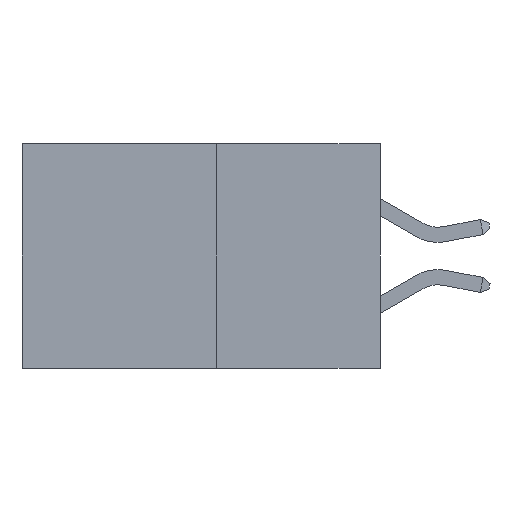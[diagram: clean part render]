
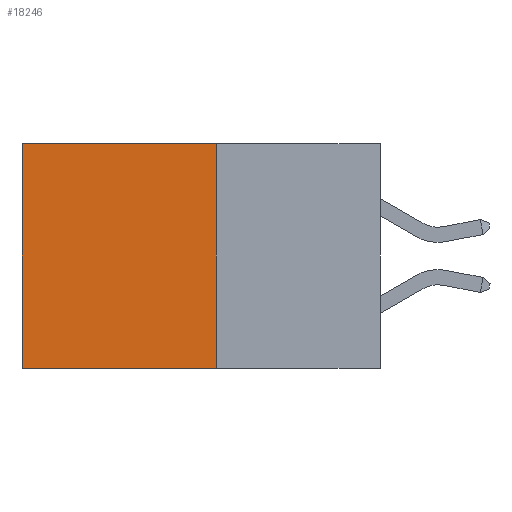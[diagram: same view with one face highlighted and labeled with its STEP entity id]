
A CAD part, left-side view. The second image highlights one B-rep face of the part: STEP entity #18246.
In plain terms, the highlighted planar face has unit normal (-1, 0, 0).
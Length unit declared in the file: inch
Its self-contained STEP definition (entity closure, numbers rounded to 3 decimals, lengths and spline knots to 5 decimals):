
#338 = CARTESIAN_POINT ( 'NONE',  ( 0.277, 0.27, -0.37 ) ) ;
#500 = CARTESIAN_POINT ( 'NONE',  ( 0.277, 0.27, 0. ) ) ;
#790 = VERTEX_POINT ( 'NONE', #1906 ) ;
#957 = EDGE_CURVE ( 'NONE', #18103, #5772, #1752, .T. ) ;
#1347 = ORIENTED_EDGE ( 'NONE', *, *, #20250, .T. ) ;
#1752 = LINE ( 'NONE', #20085, #15234 ) ;
#1906 = CARTESIAN_POINT ( 'NONE',  ( 0.277, 0.59, 0. ) ) ;
#2418 = EDGE_CURVE ( 'NONE', #790, #13445, #4125, .T. ) ;
#2867 = DIRECTION ( 'NONE',  ( 0., 1., 0. ) ) ;
#2894 = ORIENTED_EDGE ( 'NONE', *, *, #2418, .T. ) ;
#4125 = LINE ( 'NONE', #16833, #8122 ) ;
#4263 = DIRECTION ( 'NONE',  ( 1., 0., 0. ) ) ;
#5726 = CARTESIAN_POINT ( 'NONE',  ( 0.277, 0.59, -0.37 ) ) ;
#5772 = VERTEX_POINT ( 'NONE', #12422 ) ;
#5781 = ORIENTED_EDGE ( 'NONE', *, *, #957, .F. ) ;
#6367 = LINE ( 'NONE', #11327, #10371 ) ;
#6888 = DIRECTION ( 'NONE',  ( 0., 0., -1. ) ) ;
#7282 = FACE_OUTER_BOUND ( 'NONE', #9623, .T. ) ;
#8122 = VECTOR ( 'NONE', #15710, 39.37008 ) ;
#9623 = EDGE_LOOP ( 'NONE', ( #2894, #12051, #5781, #1347 ) ) ;
#9779 = EDGE_CURVE ( 'NONE', #5772, #13445, #17468, .T. ) ;
#10371 = VECTOR ( 'NONE', #2867, 39.37008 ) ;
#11028 = PLANE ( 'NONE',  #14331 ) ;
#11327 = CARTESIAN_POINT ( 'NONE',  ( 0.277, 0.27, 0. ) ) ;
#12051 = ORIENTED_EDGE ( 'NONE', *, *, #9779, .F. ) ;
#12422 = CARTESIAN_POINT ( 'NONE',  ( 0.277, 0.27, -0.37 ) ) ;
#13025 = VECTOR ( 'NONE', #15530, 39.37008 ) ;
#13445 = VERTEX_POINT ( 'NONE', #5726 ) ;
#14331 = AXIS2_PLACEMENT_3D ( 'NONE', #14394, #4263, #16062 ) ;
#14394 = CARTESIAN_POINT ( 'NONE',  ( 0.277, 0.27, -0.37 ) ) ;
#15234 = VECTOR ( 'NONE', #6888, 39.37008 ) ;
#15530 = DIRECTION ( 'NONE',  ( 0., 1., 0. ) ) ;
#15710 = DIRECTION ( 'NONE',  ( 0., 0., -1. ) ) ;
#16062 = DIRECTION ( 'NONE',  ( 0., 0., -1. ) ) ;
#16833 = CARTESIAN_POINT ( 'NONE',  ( 0.277, 0.59, -0.37 ) ) ;
#17468 = LINE ( 'NONE', #338, #13025 ) ;
#18103 = VERTEX_POINT ( 'NONE', #500 ) ;
#18246 = ADVANCED_FACE ( 'NONE', ( #7282 ), #11028, .F. ) ;
#20085 = CARTESIAN_POINT ( 'NONE',  ( 0.277, 0.27, -0.37 ) ) ;
#20250 = EDGE_CURVE ( 'NONE', #18103, #790, #6367, .T. ) ;
